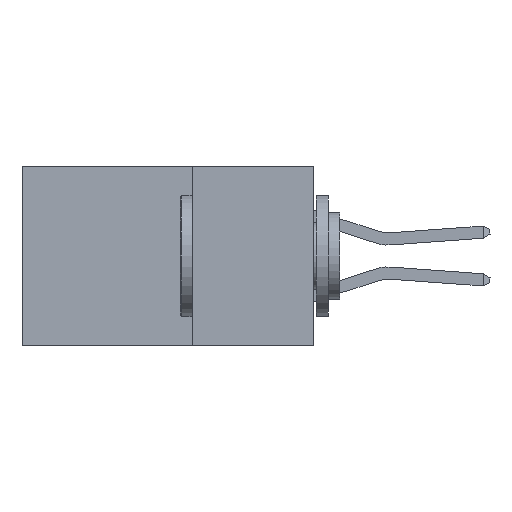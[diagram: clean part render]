
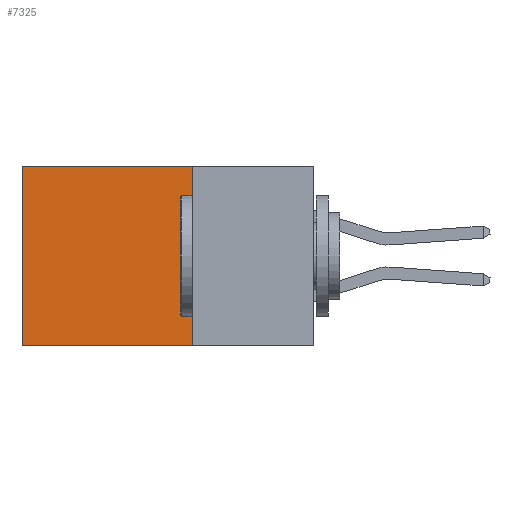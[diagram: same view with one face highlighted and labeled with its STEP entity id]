
A CAD part, left-side view. The second image highlights one B-rep face of the part: STEP entity #7325.
In plain terms, the highlighted planar face has unit normal (-1, 0, 0).
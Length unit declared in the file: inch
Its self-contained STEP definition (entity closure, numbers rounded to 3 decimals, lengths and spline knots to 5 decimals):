
#762 = CARTESIAN_POINT ( 'NONE',  ( 0.2875, 0.25, -0.37 ) ) ;
#835 = EDGE_CURVE ( 'NONE', #5093, #10077, #4677, .T. ) ;
#1377 = ORIENTED_EDGE ( 'NONE', *, *, #1713, .T. ) ;
#1648 = DIRECTION ( 'NONE',  ( 1., 0., 0. ) ) ;
#1682 = AXIS2_PLACEMENT_3D ( 'NONE', #5487, #1648, #8353 ) ;
#1713 = EDGE_CURVE ( 'NONE', #9913, #2561, #7472, .T. ) ;
#1715 = ORIENTED_EDGE ( 'NONE', *, *, #11124, .T. ) ;
#1846 = DIRECTION ( 'NONE',  ( 0., 1., 0. ) ) ;
#2545 = CARTESIAN_POINT ( 'NONE',  ( 0.2875, 0.6, 0. ) ) ;
#2561 = VERTEX_POINT ( 'NONE', #11666 ) ;
#2686 = VECTOR ( 'NONE', #1846, 39.37008 ) ;
#2913 = CARTESIAN_POINT ( 'NONE',  ( 0.2875, 0.6, 0. ) ) ;
#3056 = VECTOR ( 'NONE', #12224, 39.37008 ) ;
#3436 = LINE ( 'NONE', #3898, #8410 ) ;
#3898 = CARTESIAN_POINT ( 'NONE',  ( 0.2875, 0.25, 0. ) ) ;
#4677 = LINE ( 'NONE', #9816, #4951 ) ;
#4797 = DIRECTION ( 'NONE',  ( 0., 1., 0. ) ) ;
#4951 = VECTOR ( 'NONE', #5682, 39.37008 ) ;
#5093 = VERTEX_POINT ( 'NONE', #7482 ) ;
#5487 = CARTESIAN_POINT ( 'NONE',  ( 0.2875, 0.25, 0. ) ) ;
#5682 = DIRECTION ( 'NONE',  ( 0., 0., -1. ) ) ;
#5757 = LINE ( 'NONE', #762, #2686 ) ;
#6997 = CARTESIAN_POINT ( 'NONE',  ( 0.2875, 0.25, -0.37 ) ) ;
#7325 = ADVANCED_FACE ( 'NONE', ( #11920 ), #7430, .F. ) ;
#7430 = PLANE ( 'NONE',  #1682 ) ;
#7472 = LINE ( 'NONE', #2545, #3056 ) ;
#7482 = CARTESIAN_POINT ( 'NONE',  ( 0.2875, 0.25, 0. ) ) ;
#8353 = DIRECTION ( 'NONE',  ( 0., 0., -1. ) ) ;
#8410 = VECTOR ( 'NONE', #4797, 39.37008 ) ;
#9012 = ORIENTED_EDGE ( 'NONE', *, *, #10493, .F. ) ;
#9663 = EDGE_LOOP ( 'NONE', ( #1377, #9012, #11341, #1715 ) ) ;
#9816 = CARTESIAN_POINT ( 'NONE',  ( 0.2875, 0.25, 0. ) ) ;
#9913 = VERTEX_POINT ( 'NONE', #2913 ) ;
#10077 = VERTEX_POINT ( 'NONE', #6997 ) ;
#10493 = EDGE_CURVE ( 'NONE', #10077, #2561, #5757, .T. ) ;
#11124 = EDGE_CURVE ( 'NONE', #5093, #9913, #3436, .T. ) ;
#11341 = ORIENTED_EDGE ( 'NONE', *, *, #835, .F. ) ;
#11666 = CARTESIAN_POINT ( 'NONE',  ( 0.2875, 0.6, -0.37 ) ) ;
#11920 = FACE_OUTER_BOUND ( 'NONE', #9663, .T. ) ;
#12224 = DIRECTION ( 'NONE',  ( 0., 0., -1. ) ) ;
